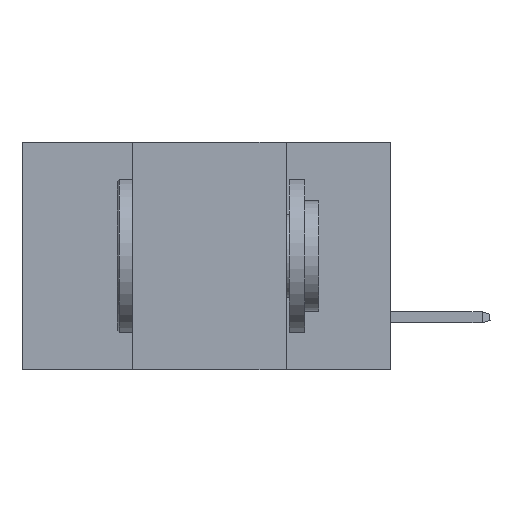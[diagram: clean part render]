
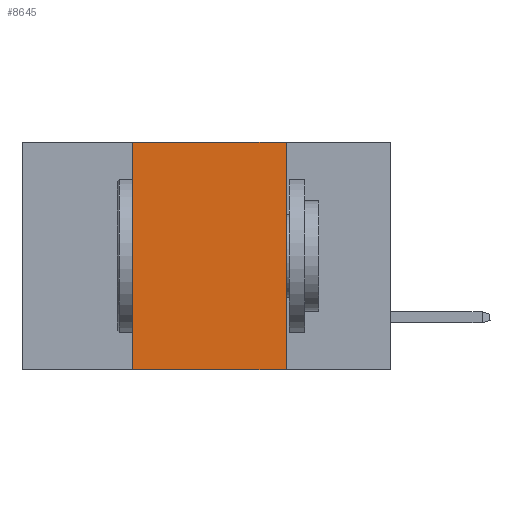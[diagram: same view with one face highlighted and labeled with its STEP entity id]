
A CAD part, left-side view. The second image highlights one B-rep face of the part: STEP entity #8645.
In plain terms, the highlighted planar face has unit normal (-1, 0, 0).
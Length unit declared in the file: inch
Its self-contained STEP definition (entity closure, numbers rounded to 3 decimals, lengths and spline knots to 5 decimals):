
#456 = LINE ( 'NONE', #9452, #10154 ) ;
#5597 = EDGE_CURVE ( 'NONE', #25694, #16332, #19874, .T. ) ;
#5921 = AXIS2_PLACEMENT_3D ( 'NONE', #12837, #30114, #13160 ) ;
#6491 = CARTESIAN_POINT ( 'NONE',  ( 0., 0.42, 0. ) ) ;
#8484 = EDGE_CURVE ( 'NONE', #28494, #11857, #26328, .T. ) ;
#8645 = ADVANCED_FACE ( 'NONE', ( #31222 ), #10584, .F. ) ;
#9090 = CARTESIAN_POINT ( 'NONE',  ( 0., 0.42, -0.37 ) ) ;
#9452 = CARTESIAN_POINT ( 'NONE',  ( 0., 0.6, -0.37 ) ) ;
#10154 = VECTOR ( 'NONE', #13999, 39.37008 ) ;
#10320 = CARTESIAN_POINT ( 'NONE',  ( 0., 0.17, 0. ) ) ;
#10584 = PLANE ( 'NONE',  #5921 ) ;
#11400 = DIRECTION ( 'NONE',  ( 0., -1., 0. ) ) ;
#11857 = VERTEX_POINT ( 'NONE', #6491 ) ;
#12001 = LINE ( 'NONE', #13765, #26617 ) ;
#12837 = CARTESIAN_POINT ( 'NONE',  ( 0., 0.6, 0. ) ) ;
#13160 = DIRECTION ( 'NONE',  ( 0., 0., -1. ) ) ;
#13765 = CARTESIAN_POINT ( 'NONE',  ( 0., 0.6, 0. ) ) ;
#13885 = ORIENTED_EDGE ( 'NONE', *, *, #28330, .F. ) ;
#13999 = DIRECTION ( 'NONE',  ( 0., -1., 0. ) ) ;
#15461 = EDGE_LOOP ( 'NONE', ( #19829, #13885, #28003, #22681 ) ) ;
#15513 = VECTOR ( 'NONE', #19323, 39.37008 ) ;
#16332 = VERTEX_POINT ( 'NONE', #18233 ) ;
#18233 = CARTESIAN_POINT ( 'NONE',  ( 0., 0.17, -0.37 ) ) ;
#19095 = CARTESIAN_POINT ( 'NONE',  ( 0., 0.17, 0. ) ) ;
#19323 = DIRECTION ( 'NONE',  ( 0., 0., 1. ) ) ;
#19829 = ORIENTED_EDGE ( 'NONE', *, *, #5597, .F. ) ;
#19874 = LINE ( 'NONE', #10320, #20258 ) ;
#20185 = DIRECTION ( 'NONE',  ( 0., 0., -1. ) ) ;
#20258 = VECTOR ( 'NONE', #20185, 39.37008 ) ;
#21676 = CARTESIAN_POINT ( 'NONE',  ( 0., 0.42, 0. ) ) ;
#22681 = ORIENTED_EDGE ( 'NONE', *, *, #22704, .T. ) ;
#22704 = EDGE_CURVE ( 'NONE', #28494, #16332, #456, .T. ) ;
#25694 = VERTEX_POINT ( 'NONE', #19095 ) ;
#26328 = LINE ( 'NONE', #21676, #15513 ) ;
#26617 = VECTOR ( 'NONE', #11400, 39.37008 ) ;
#28003 = ORIENTED_EDGE ( 'NONE', *, *, #8484, .F. ) ;
#28330 = EDGE_CURVE ( 'NONE', #11857, #25694, #12001, .T. ) ;
#28494 = VERTEX_POINT ( 'NONE', #9090 ) ;
#30114 = DIRECTION ( 'NONE',  ( 1., 0., 0. ) ) ;
#31222 = FACE_OUTER_BOUND ( 'NONE', #15461, .T. ) ;
